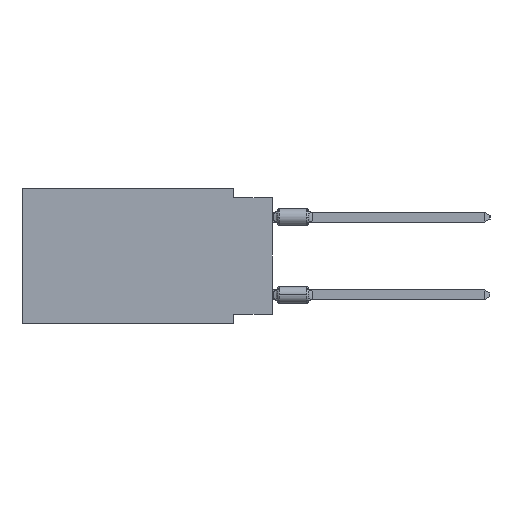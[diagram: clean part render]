
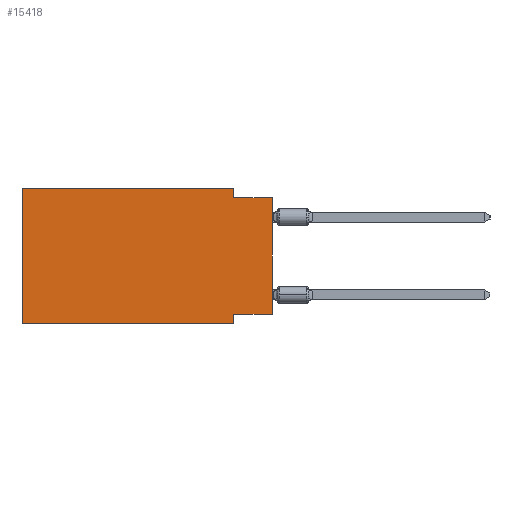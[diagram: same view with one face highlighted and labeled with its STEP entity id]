
A CAD part, left-side view. The second image highlights one B-rep face of the part: STEP entity #15418.
In plain terms, the highlighted planar face has unit normal (-1, 0, 0).
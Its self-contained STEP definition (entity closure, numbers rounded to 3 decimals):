
#221 = CARTESIAN_POINT ( 'NONE',  ( 0., 2.54, 0. ) ) ;
#912 = ORIENTED_EDGE ( 'NONE', *, *, #7653, .F. ) ;
#6617 = VECTOR ( 'NONE', #11107, 1000. ) ;
#7653 = EDGE_CURVE ( 'NONE', #59742, #42790, #52733, .T. ) ;
#8911 = EDGE_CURVE ( 'NONE', #15030, #9785, #58467, .T. ) ;
#9785 = VERTEX_POINT ( 'NONE', #17651 ) ;
#10123 = CARTESIAN_POINT ( 'NONE',  ( 0., 0., -0.635 ) ) ;
#11107 = DIRECTION ( 'NONE',  ( 0., 0., -1. ) ) ;
#11304 = EDGE_CURVE ( 'NONE', #59742, #35565, #57676, .T. ) ;
#12100 = DIRECTION ( 'NONE',  ( 0., 0., -1. ) ) ;
#14150 = VECTOR ( 'NONE', #61118, 1000. ) ;
#15030 = VERTEX_POINT ( 'NONE', #221 ) ;
#15221 = LINE ( 'NONE', #30902, #6617 ) ;
#15418 = ADVANCED_FACE ( 'NONE', ( #64080 ), #17403, .F. ) ;
#17403 = PLANE ( 'NONE',  #43763 ) ;
#17555 = CARTESIAN_POINT ( 'NONE',  ( 0., 2.54, 0. ) ) ;
#17651 = CARTESIAN_POINT ( 'NONE',  ( 0., 2.54, -0.635 ) ) ;
#20029 = LINE ( 'NONE', #66021, #54914 ) ;
#20329 = VECTOR ( 'NONE', #12100, 1000. ) ;
#21110 = VERTEX_POINT ( 'NONE', #51894 ) ;
#22811 = CARTESIAN_POINT ( 'NONE',  ( 0., 16.383, -8.89 ) ) ;
#23506 = DIRECTION ( 'NONE',  ( 0., -1., 0. ) ) ;
#23553 = VECTOR ( 'NONE', #55744, 1000. ) ;
#28301 = DIRECTION ( 'NONE',  ( 1., 0., 0. ) ) ;
#29225 = ORIENTED_EDGE ( 'NONE', *, *, #59947, .F. ) ;
#30538 = CARTESIAN_POINT ( 'NONE',  ( 0., 16.383, 0. ) ) ;
#30902 = CARTESIAN_POINT ( 'NONE',  ( 0., 2.54, -8.89 ) ) ;
#32113 = DIRECTION ( 'NONE',  ( 0., -1., 0. ) ) ;
#35565 = VERTEX_POINT ( 'NONE', #64607 ) ;
#37603 = EDGE_CURVE ( 'NONE', #42790, #15030, #49406, .T. ) ;
#37621 = ORIENTED_EDGE ( 'NONE', *, *, #39801, .F. ) ;
#38045 = DIRECTION ( 'NONE',  ( 0., 0., 1. ) ) ;
#38083 = ORIENTED_EDGE ( 'NONE', *, *, #37603, .F. ) ;
#38164 = DIRECTION ( 'NONE',  ( 0., 0., -1. ) ) ;
#39480 = ORIENTED_EDGE ( 'NONE', *, *, #63523, .F. ) ;
#39801 = EDGE_CURVE ( 'NONE', #48705, #35565, #15221, .T. ) ;
#40269 = VECTOR ( 'NONE', #32113, 1000. ) ;
#40749 = LINE ( 'NONE', #67323, #23553 ) ;
#41045 = EDGE_CURVE ( 'NONE', #21110, #59961, #40749, .T. ) ;
#42790 = VERTEX_POINT ( 'NONE', #30538 ) ;
#42952 = CARTESIAN_POINT ( 'NONE',  ( 0., 16.383, 0. ) ) ;
#43763 = AXIS2_PLACEMENT_3D ( 'NONE', #42952, #28301, #38164 ) ;
#44270 = CARTESIAN_POINT ( 'NONE',  ( 0., 16.383, 0. ) ) ;
#47281 = CARTESIAN_POINT ( 'NONE',  ( 0., 16.383, 0. ) ) ;
#47391 = EDGE_LOOP ( 'NONE', ( #57552, #29225, #57691, #38083, #912, #59049, #37621, #39480 ) ) ;
#47781 = VECTOR ( 'NONE', #23506, 1000. ) ;
#48705 = VERTEX_POINT ( 'NONE', #54058 ) ;
#49406 = LINE ( 'NONE', #44270, #47781 ) ;
#51894 = CARTESIAN_POINT ( 'NONE',  ( 0., 0., -8.255 ) ) ;
#52733 = LINE ( 'NONE', #47281, #63700 ) ;
#54058 = CARTESIAN_POINT ( 'NONE',  ( 0., 2.54, -8.255 ) ) ;
#54914 = VECTOR ( 'NONE', #66356, 1000. ) ;
#55744 = DIRECTION ( 'NONE',  ( 0., 0., 1. ) ) ;
#56011 = LINE ( 'NONE', #66565, #14150 ) ;
#57552 = ORIENTED_EDGE ( 'NONE', *, *, #41045, .T. ) ;
#57676 = LINE ( 'NONE', #62113, #40269 ) ;
#57691 = ORIENTED_EDGE ( 'NONE', *, *, #8911, .F. ) ;
#58467 = LINE ( 'NONE', #17555, #20329 ) ;
#59049 = ORIENTED_EDGE ( 'NONE', *, *, #11304, .T. ) ;
#59742 = VERTEX_POINT ( 'NONE', #22811 ) ;
#59947 = EDGE_CURVE ( 'NONE', #9785, #59961, #20029, .T. ) ;
#59961 = VERTEX_POINT ( 'NONE', #10123 ) ;
#61118 = DIRECTION ( 'NONE',  ( 0., 1., 0. ) ) ;
#62113 = CARTESIAN_POINT ( 'NONE',  ( 0., 16.383, -8.89 ) ) ;
#63523 = EDGE_CURVE ( 'NONE', #21110, #48705, #56011, .T. ) ;
#63700 = VECTOR ( 'NONE', #38045, 1000. ) ;
#64080 = FACE_OUTER_BOUND ( 'NONE', #47391, .T. ) ;
#64607 = CARTESIAN_POINT ( 'NONE',  ( 0., 2.54, -8.89 ) ) ;
#66021 = CARTESIAN_POINT ( 'NONE',  ( 0., 0., -0.635 ) ) ;
#66356 = DIRECTION ( 'NONE',  ( 0., -1., 0. ) ) ;
#66565 = CARTESIAN_POINT ( 'NONE',  ( 0., 0., -8.255 ) ) ;
#67323 = CARTESIAN_POINT ( 'NONE',  ( 0., 0., 0. ) ) ;
